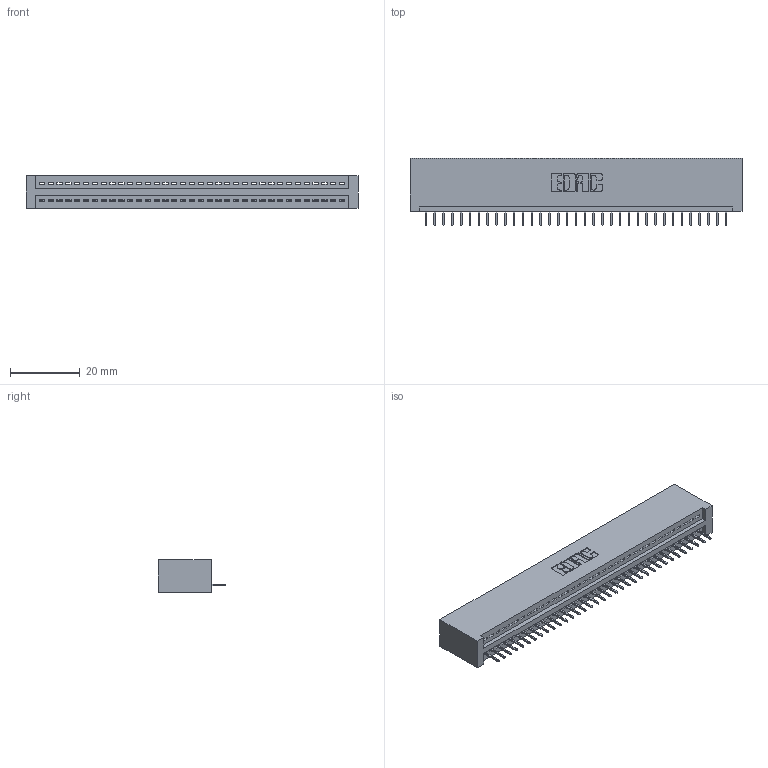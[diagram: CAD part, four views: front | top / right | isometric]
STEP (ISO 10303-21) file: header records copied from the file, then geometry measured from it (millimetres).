
FILE_DESCRIPTION (( 'STEP AP203' ), '1' );
FILE_NAME ('345-035-524-101.STEP', '2019-10-07T20:48:05', ( '' ), ( '' ), 'SwSTEP 2.0', 'SolidWorks 2016', '' );
FILE_SCHEMA (( 'CONFIG_CONTROL_DESIGN' ));
Length unit declared in the file: inch
Products named in the file (3): 345-035-524-101; 345 Part_No Mounting Lugs; 345-292-001_345-293-124
Assembly tree (36 placements, depth 2):
  345-035-524-101
    345 Part_No Mounting Lugs
    345-292-001_345-293-124  x35
Bounding box: 95.5 x 19.35 x 9.4 mm (x, y, z)
Volume: 9459.8 mm3; surface area: 12224.2 mm2
Topology: 36 solids, 36 shells, 2288 faces, 6617 edges, 4270 vertices
Faces by surface type: plane 1686, cylinder 602
Entity records: 27081 total; most frequent: CARTESIAN_POINT 4697, ORIENTED_EDGE 4666, DIRECTION 4107, EDGE_CURVE 2333, VECTOR 2073, LINE 2073, VERTEX_POINT 1550, AXIS2_PLACEMENT_3D 1017
